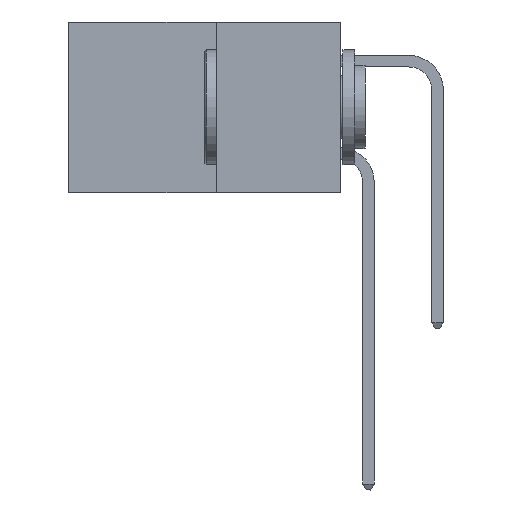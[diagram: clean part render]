
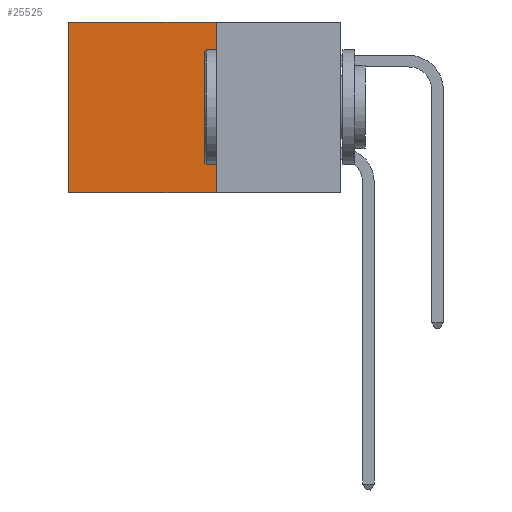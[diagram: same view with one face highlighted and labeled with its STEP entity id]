
A CAD part, left-side view. The second image highlights one B-rep face of the part: STEP entity #25525.
In plain terms, the highlighted planar face has unit normal (-1, 0, 0).
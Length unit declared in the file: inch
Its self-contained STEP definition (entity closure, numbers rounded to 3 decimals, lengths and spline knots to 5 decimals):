
#1105 = CARTESIAN_POINT ( 'NONE',  ( 0.277, 0.59, 0. ) ) ;
#1500 = CARTESIAN_POINT ( 'NONE',  ( 0.277, 0.59, -0.37 ) ) ;
#2294 = CARTESIAN_POINT ( 'NONE',  ( 0.277, 0.27, -0.37 ) ) ;
#2955 = CARTESIAN_POINT ( 'NONE',  ( 0.277, 0.59, -0.37 ) ) ;
#3282 = VECTOR ( 'NONE', #12075, 39.37008 ) ;
#3538 = ORIENTED_EDGE ( 'NONE', *, *, #7445, .T. ) ;
#3999 = LINE ( 'NONE', #2955, #3282 ) ;
#4582 = DIRECTION ( 'NONE',  ( 0., 0., -1. ) ) ;
#4777 = LINE ( 'NONE', #23013, #16148 ) ;
#5144 = LINE ( 'NONE', #5601, #16521 ) ;
#5601 = CARTESIAN_POINT ( 'NONE',  ( 0.277, 0.27, -0.37 ) ) ;
#7408 = VERTEX_POINT ( 'NONE', #27860 ) ;
#7445 = EDGE_CURVE ( 'NONE', #8295, #8438, #3999, .T. ) ;
#8013 = EDGE_CURVE ( 'NONE', #7408, #8295, #24596, .T. ) ;
#8295 = VERTEX_POINT ( 'NONE', #1105 ) ;
#8438 = VERTEX_POINT ( 'NONE', #1500 ) ;
#9296 = CARTESIAN_POINT ( 'NONE',  ( 0.277, 0.27, 0. ) ) ;
#10077 = DIRECTION ( 'NONE',  ( 0., 0., -1. ) ) ;
#11325 = PLANE ( 'NONE',  #24723 ) ;
#11552 = EDGE_CURVE ( 'NONE', #7408, #13468, #5144, .T. ) ;
#11765 = VECTOR ( 'NONE', #18448, 39.37008 ) ;
#12075 = DIRECTION ( 'NONE',  ( 0., 0., -1. ) ) ;
#12269 = ORIENTED_EDGE ( 'NONE', *, *, #8013, .T. ) ;
#13468 = VERTEX_POINT ( 'NONE', #28579 ) ;
#13501 = EDGE_LOOP ( 'NONE', ( #3538, #13888, #25983, #12269 ) ) ;
#13888 = ORIENTED_EDGE ( 'NONE', *, *, #17824, .F. ) ;
#16148 = VECTOR ( 'NONE', #25311, 39.37008 ) ;
#16521 = VECTOR ( 'NONE', #10077, 39.37008 ) ;
#17824 = EDGE_CURVE ( 'NONE', #13468, #8438, #4777, .T. ) ;
#18222 = DIRECTION ( 'NONE',  ( 1., 0., 0. ) ) ;
#18448 = DIRECTION ( 'NONE',  ( 0., 1., 0. ) ) ;
#23013 = CARTESIAN_POINT ( 'NONE',  ( 0.277, 0.27, -0.37 ) ) ;
#24596 = LINE ( 'NONE', #9296, #11765 ) ;
#24723 = AXIS2_PLACEMENT_3D ( 'NONE', #2294, #18222, #4582 ) ;
#25311 = DIRECTION ( 'NONE',  ( 0., 1., 0. ) ) ;
#25525 = ADVANCED_FACE ( 'NONE', ( #26904 ), #11325, .F. ) ;
#25983 = ORIENTED_EDGE ( 'NONE', *, *, #11552, .F. ) ;
#26904 = FACE_OUTER_BOUND ( 'NONE', #13501, .T. ) ;
#27860 = CARTESIAN_POINT ( 'NONE',  ( 0.277, 0.27, 0. ) ) ;
#28579 = CARTESIAN_POINT ( 'NONE',  ( 0.277, 0.27, -0.37 ) ) ;
